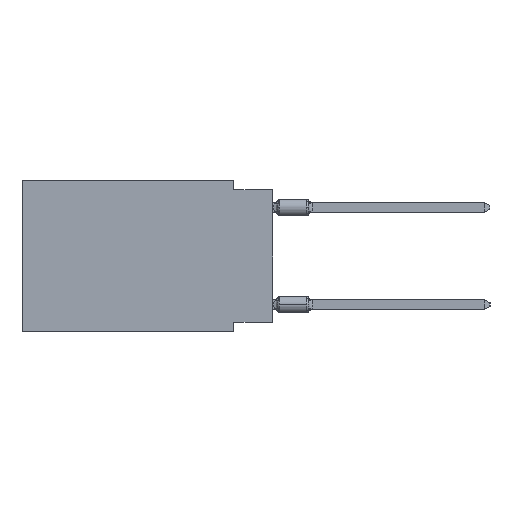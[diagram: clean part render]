
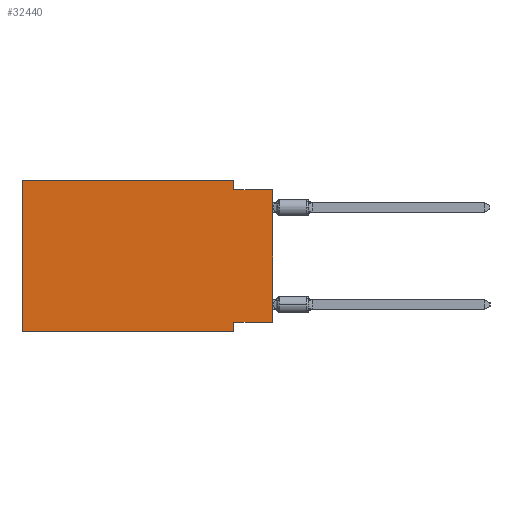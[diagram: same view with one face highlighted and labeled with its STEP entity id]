
A CAD part, left-side view. The second image highlights one B-rep face of the part: STEP entity #32440.
In plain terms, the highlighted planar face has unit normal (-1, 0, 0).
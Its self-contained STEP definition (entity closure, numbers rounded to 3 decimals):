
#995 = DIRECTION ( 'NONE',  ( 0., 1., 0. ) ) ;
#2987 = LINE ( 'NONE', #19922, #30052 ) ;
#3400 = CARTESIAN_POINT ( 'NONE',  ( 0., 16.383, 0. ) ) ;
#4379 = CARTESIAN_POINT ( 'NONE',  ( 0., 16.383, 0. ) ) ;
#4707 = LINE ( 'NONE', #25290, #10164 ) ;
#4759 = DIRECTION ( 'NONE',  ( 0., 0., 1. ) ) ;
#5975 = ORIENTED_EDGE ( 'NONE', *, *, #14668, .T. ) ;
#6475 = LINE ( 'NONE', #27284, #44571 ) ;
#6635 = DIRECTION ( 'NONE',  ( 0., 0., -1. ) ) ;
#6688 = DIRECTION ( 'NONE',  ( 0., -1., 0. ) ) ;
#7375 = EDGE_CURVE ( 'NONE', #44991, #36879, #6475, .T. ) ;
#8210 = CARTESIAN_POINT ( 'NONE',  ( 0., 2.54, -9.906 ) ) ;
#8430 = ORIENTED_EDGE ( 'NONE', *, *, #12668, .F. ) ;
#8995 = EDGE_CURVE ( 'NONE', #19703, #36879, #2987, .T. ) ;
#9705 = EDGE_CURVE ( 'NONE', #44991, #41942, #33075, .T. ) ;
#10164 = VECTOR ( 'NONE', #11355, 1000. ) ;
#11195 = ORIENTED_EDGE ( 'NONE', *, *, #8995, .F. ) ;
#11355 = DIRECTION ( 'NONE',  ( 0., -1., 0. ) ) ;
#11421 = DIRECTION ( 'NONE',  ( 0., 0., -1. ) ) ;
#12668 = EDGE_CURVE ( 'NONE', #41942, #17144, #34727, .T. ) ;
#13158 = DIRECTION ( 'NONE',  ( 0., 0., -1. ) ) ;
#14106 = EDGE_CURVE ( 'NONE', #30922, #30410, #4707, .T. ) ;
#14233 = CARTESIAN_POINT ( 'NONE',  ( 0., 2.54, 0. ) ) ;
#14668 = EDGE_CURVE ( 'NONE', #40005, #30410, #22681, .T. ) ;
#15206 = CARTESIAN_POINT ( 'NONE',  ( 0., 0., -9.271 ) ) ;
#15954 = VECTOR ( 'NONE', #27619, 1000. ) ;
#16609 = FACE_OUTER_BOUND ( 'NONE', #37559, .T. ) ;
#16698 = CARTESIAN_POINT ( 'NONE',  ( 0., 0., -0.635 ) ) ;
#17144 = VERTEX_POINT ( 'NONE', #14233 ) ;
#17597 = VECTOR ( 'NONE', #995, 1000. ) ;
#18241 = VECTOR ( 'NONE', #40520, 1000. ) ;
#18705 = CARTESIAN_POINT ( 'NONE',  ( 0., 16.383, 0. ) ) ;
#19029 = LINE ( 'NONE', #42609, #17597 ) ;
#19703 = VERTEX_POINT ( 'NONE', #40850 ) ;
#19922 = CARTESIAN_POINT ( 'NONE',  ( 0., 2.54, -9.906 ) ) ;
#21602 = EDGE_CURVE ( 'NONE', #40005, #19703, #19029, .T. ) ;
#21992 = CARTESIAN_POINT ( 'NONE',  ( 0., 16.383, -9.906 ) ) ;
#22681 = LINE ( 'NONE', #36624, #18241 ) ;
#24468 = ORIENTED_EDGE ( 'NONE', *, *, #9705, .F. ) ;
#24633 = CARTESIAN_POINT ( 'NONE',  ( 0., 2.54, -0.635 ) ) ;
#25290 = CARTESIAN_POINT ( 'NONE',  ( 0., 0., -0.635 ) ) ;
#26204 = CARTESIAN_POINT ( 'NONE',  ( 0., 16.383, 0. ) ) ;
#27284 = CARTESIAN_POINT ( 'NONE',  ( 0., 16.383, -9.906 ) ) ;
#27619 = DIRECTION ( 'NONE',  ( 0., -1., 0. ) ) ;
#28790 = LINE ( 'NONE', #42733, #41273 ) ;
#30052 = VECTOR ( 'NONE', #6635, 1000. ) ;
#30200 = ORIENTED_EDGE ( 'NONE', *, *, #14106, .F. ) ;
#30316 = PLANE ( 'NONE',  #33858 ) ;
#30410 = VERTEX_POINT ( 'NONE', #16698 ) ;
#30535 = DIRECTION ( 'NONE',  ( 1., 0., 0. ) ) ;
#30922 = VERTEX_POINT ( 'NONE', #24633 ) ;
#32440 = ADVANCED_FACE ( 'NONE', ( #16609 ), #30316, .F. ) ;
#33075 = LINE ( 'NONE', #18705, #43237 ) ;
#33858 = AXIS2_PLACEMENT_3D ( 'NONE', #26204, #30535, #13158 ) ;
#34467 = ORIENTED_EDGE ( 'NONE', *, *, #21602, .F. ) ;
#34727 = LINE ( 'NONE', #3400, #15954 ) ;
#36361 = ORIENTED_EDGE ( 'NONE', *, *, #37741, .F. ) ;
#36624 = CARTESIAN_POINT ( 'NONE',  ( 0., 0., 0. ) ) ;
#36879 = VERTEX_POINT ( 'NONE', #8210 ) ;
#37559 = EDGE_LOOP ( 'NONE', ( #5975, #30200, #36361, #8430, #24468, #40825, #11195, #34467 ) ) ;
#37741 = EDGE_CURVE ( 'NONE', #17144, #30922, #28790, .T. ) ;
#40005 = VERTEX_POINT ( 'NONE', #15206 ) ;
#40520 = DIRECTION ( 'NONE',  ( 0., 0., 1. ) ) ;
#40825 = ORIENTED_EDGE ( 'NONE', *, *, #7375, .T. ) ;
#40850 = CARTESIAN_POINT ( 'NONE',  ( 0., 2.54, -9.271 ) ) ;
#41273 = VECTOR ( 'NONE', #11421, 1000. ) ;
#41942 = VERTEX_POINT ( 'NONE', #4379 ) ;
#42609 = CARTESIAN_POINT ( 'NONE',  ( 0., 0., -9.271 ) ) ;
#42733 = CARTESIAN_POINT ( 'NONE',  ( 0., 2.54, 0. ) ) ;
#43237 = VECTOR ( 'NONE', #4759, 1000. ) ;
#44571 = VECTOR ( 'NONE', #6688, 1000. ) ;
#44991 = VERTEX_POINT ( 'NONE', #21992 ) ;
